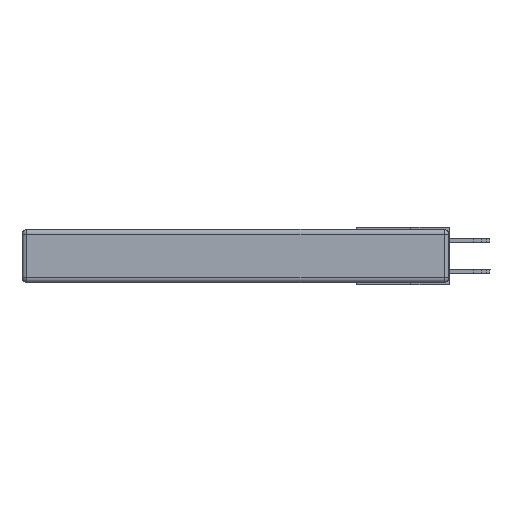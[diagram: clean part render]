
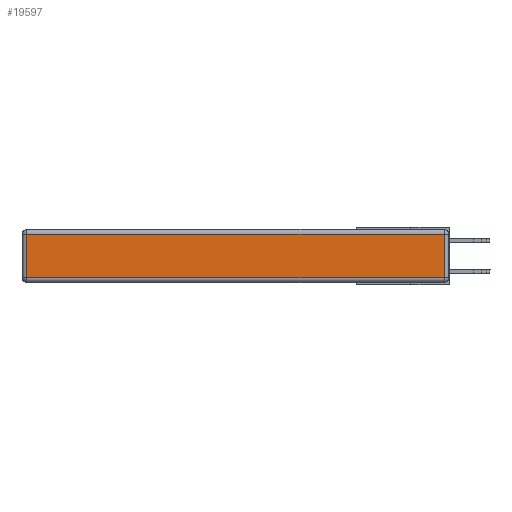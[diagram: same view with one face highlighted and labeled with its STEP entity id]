
A CAD part, left-side view. The second image highlights one B-rep face of the part: STEP entity #19597.
In plain terms, the highlighted planar face has unit normal (-1, 0, 0).
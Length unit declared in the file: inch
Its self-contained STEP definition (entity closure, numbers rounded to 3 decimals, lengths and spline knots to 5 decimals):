
#200 = CARTESIAN_POINT ( 'NONE',  ( 0., 0., -0.313 ) ) ;
#1055 = DIRECTION ( 'NONE',  ( 0., 0., -1. ) ) ;
#1207 = CARTESIAN_POINT ( 'NONE',  ( 0., 0.03, -0.313 ) ) ;
#1542 = CARTESIAN_POINT ( 'NONE',  ( 0., 0., -0.343 ) ) ;
#1680 = PLANE ( 'NONE',  #18237 ) ;
#2056 = EDGE_CURVE ( 'NONE', #13395, #17318, #4789, .T. ) ;
#3096 = DIRECTION ( 'NONE',  ( 0., 1., 0. ) ) ;
#3152 = DIRECTION ( 'NONE',  ( 0., 0., 1. ) ) ;
#3353 = ORIENTED_EDGE ( 'NONE', *, *, #2056, .T. ) ;
#3426 = VECTOR ( 'NONE', #6652, 39.37008 ) ;
#3472 = EDGE_CURVE ( 'NONE', #15518, #12455, #13332, .T. ) ;
#3664 = LINE ( 'NONE', #200, #3426 ) ;
#4789 = LINE ( 'NONE', #19803, #14818 ) ;
#5562 = ORIENTED_EDGE ( 'NONE', *, *, #12221, .T. ) ;
#6652 = DIRECTION ( 'NONE',  ( 0., -1., 0. ) ) ;
#7164 = CARTESIAN_POINT ( 'NONE',  ( 0., 2.72, -0.03 ) ) ;
#7596 = CARTESIAN_POINT ( 'NONE',  ( 0., 2.75, -0.03 ) ) ;
#8054 = DIRECTION ( 'NONE',  ( -1., 0., 0. ) ) ;
#10064 = ORIENTED_EDGE ( 'NONE', *, *, #12525, .T. ) ;
#10539 = EDGE_LOOP ( 'NONE', ( #10064, #10769, #5562, #3353 ) ) ;
#10545 = LINE ( 'NONE', #7596, #10800 ) ;
#10769 = ORIENTED_EDGE ( 'NONE', *, *, #3472, .T. ) ;
#10800 = VECTOR ( 'NONE', #3096, 39.37008 ) ;
#12221 = EDGE_CURVE ( 'NONE', #12455, #13395, #10545, .T. ) ;
#12455 = VERTEX_POINT ( 'NONE', #14454 ) ;
#12525 = EDGE_CURVE ( 'NONE', #17318, #15518, #3664, .T. ) ;
#12543 = CARTESIAN_POINT ( 'NONE',  ( 0., 2.72, -0.313 ) ) ;
#13332 = LINE ( 'NONE', #18977, #17009 ) ;
#13395 = VERTEX_POINT ( 'NONE', #7164 ) ;
#14454 = CARTESIAN_POINT ( 'NONE',  ( 0., 0.03, -0.03 ) ) ;
#14777 = FACE_OUTER_BOUND ( 'NONE', #10539, .T. ) ;
#14818 = VECTOR ( 'NONE', #1055, 39.37008 ) ;
#15518 = VERTEX_POINT ( 'NONE', #1207 ) ;
#17009 = VECTOR ( 'NONE', #17387, 39.37008 ) ;
#17318 = VERTEX_POINT ( 'NONE', #12543 ) ;
#17387 = DIRECTION ( 'NONE',  ( 0., 0., 1. ) ) ;
#18237 = AXIS2_PLACEMENT_3D ( 'NONE', #1542, #8054, #3152 ) ;
#18977 = CARTESIAN_POINT ( 'NONE',  ( 0., 0.03, -0.343 ) ) ;
#19597 = ADVANCED_FACE ( 'NONE', ( #14777 ), #1680, .T. ) ;
#19803 = CARTESIAN_POINT ( 'NONE',  ( 0., 2.72, -0.343 ) ) ;
